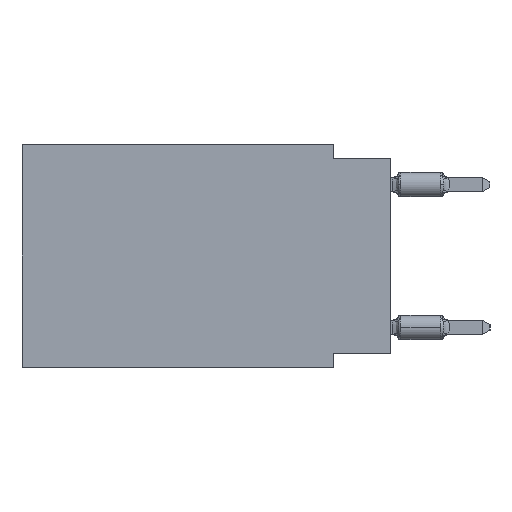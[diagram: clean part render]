
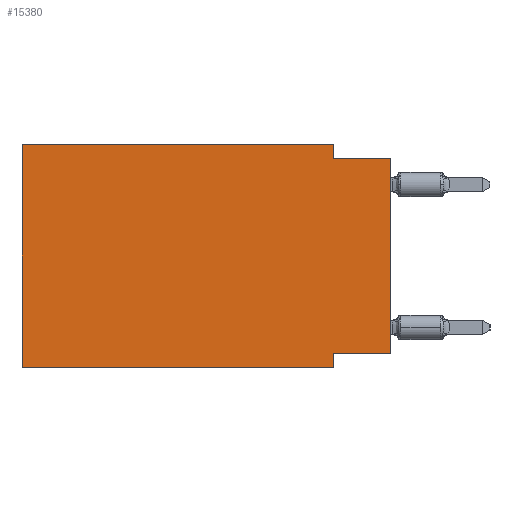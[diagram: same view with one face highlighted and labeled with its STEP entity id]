
A CAD part, left-side view. The second image highlights one B-rep face of the part: STEP entity #15380.
In plain terms, the highlighted planar face has unit normal (-1, 0, 0).
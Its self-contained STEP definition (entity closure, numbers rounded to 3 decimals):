
#7 = CARTESIAN_POINT ( 'NONE',  ( 0., 16.383, 0. ) ) ;
#449 = DIRECTION ( 'NONE',  ( 0., 0., 1. ) ) ;
#732 = CARTESIAN_POINT ( 'NONE',  ( 0., 2.54, -0.635 ) ) ;
#789 = DIRECTION ( 'NONE',  ( 0., -1., 0. ) ) ;
#908 = VECTOR ( 'NONE', #27232, 1000. ) ;
#1753 = VERTEX_POINT ( 'NONE', #9453 ) ;
#2025 = VECTOR ( 'NONE', #2217, 1000. ) ;
#2217 = DIRECTION ( 'NONE',  ( 0., 0., -1. ) ) ;
#2593 = VECTOR ( 'NONE', #26645, 1000. ) ;
#3391 = VECTOR ( 'NONE', #26401, 1000. ) ;
#3669 = VERTEX_POINT ( 'NONE', #732 ) ;
#4281 = EDGE_CURVE ( 'NONE', #1753, #36329, #9491, .T. ) ;
#4875 = CARTESIAN_POINT ( 'NONE',  ( 0., 16.383, 0. ) ) ;
#5067 = FACE_OUTER_BOUND ( 'NONE', #12217, .T. ) ;
#5641 = EDGE_CURVE ( 'NONE', #21608, #11308, #12516, .T. ) ;
#6495 = EDGE_CURVE ( 'NONE', #21608, #1753, #14164, .T. ) ;
#7492 = DIRECTION ( 'NONE',  ( 1., 0., 0. ) ) ;
#8837 = CARTESIAN_POINT ( 'NONE',  ( 0., 0., 0. ) ) ;
#9453 = CARTESIAN_POINT ( 'NONE',  ( 0., 16.383, 0. ) ) ;
#9491 = LINE ( 'NONE', #27344, #24403 ) ;
#10519 = VERTEX_POINT ( 'NONE', #10624 ) ;
#10624 = CARTESIAN_POINT ( 'NONE',  ( 0., 0., -0.635 ) ) ;
#11144 = ORIENTED_EDGE ( 'NONE', *, *, #6495, .F. ) ;
#11308 = VERTEX_POINT ( 'NONE', #15387 ) ;
#12217 = EDGE_LOOP ( 'NONE', ( #23193, #20243, #27697, #16714, #11144, #24544, #30088, #32454 ) ) ;
#12516 = LINE ( 'NONE', #26149, #17912 ) ;
#13715 = AXIS2_PLACEMENT_3D ( 'NONE', #4875, #7492, #21654 ) ;
#14164 = LINE ( 'NONE', #7, #15016 ) ;
#14856 = LINE ( 'NONE', #20455, #3391 ) ;
#14919 = CARTESIAN_POINT ( 'NONE',  ( 0., 0., -9.271 ) ) ;
#15016 = VECTOR ( 'NONE', #19937, 1000. ) ;
#15380 = ADVANCED_FACE ( 'NONE', ( #5067 ), #25196, .F. ) ;
#15387 = CARTESIAN_POINT ( 'NONE',  ( 0., 2.54, -9.906 ) ) ;
#15869 = CARTESIAN_POINT ( 'NONE',  ( 0., 2.54, 0. ) ) ;
#16714 = ORIENTED_EDGE ( 'NONE', *, *, #4281, .F. ) ;
#17912 = VECTOR ( 'NONE', #789, 1000. ) ;
#19282 = EDGE_CURVE ( 'NONE', #35319, #10519, #20199, .T. ) ;
#19937 = DIRECTION ( 'NONE',  ( 0., 0., 1. ) ) ;
#20199 = LINE ( 'NONE', #8837, #36387 ) ;
#20243 = ORIENTED_EDGE ( 'NONE', *, *, #31951, .F. ) ;
#20455 = CARTESIAN_POINT ( 'NONE',  ( 0., 0., -0.635 ) ) ;
#21068 = EDGE_CURVE ( 'NONE', #35319, #33935, #23300, .T. ) ;
#21402 = DIRECTION ( 'NONE',  ( 0., -1., 0. ) ) ;
#21608 = VERTEX_POINT ( 'NONE', #29525 ) ;
#21654 = DIRECTION ( 'NONE',  ( 0., 0., -1. ) ) ;
#22744 = CARTESIAN_POINT ( 'NONE',  ( 0., 2.54, -9.271 ) ) ;
#22899 = LINE ( 'NONE', #31072, #2025 ) ;
#23107 = EDGE_CURVE ( 'NONE', #36329, #3669, #24263, .T. ) ;
#23193 = ORIENTED_EDGE ( 'NONE', *, *, #19282, .T. ) ;
#23300 = LINE ( 'NONE', #14919, #2593 ) ;
#24034 = CARTESIAN_POINT ( 'NONE',  ( 0., 0., -9.271 ) ) ;
#24263 = LINE ( 'NONE', #15869, #908 ) ;
#24403 = VECTOR ( 'NONE', #21402, 1000. ) ;
#24544 = ORIENTED_EDGE ( 'NONE', *, *, #5641, .T. ) ;
#25196 = PLANE ( 'NONE',  #13715 ) ;
#26149 = CARTESIAN_POINT ( 'NONE',  ( 0., 16.383, -9.906 ) ) ;
#26401 = DIRECTION ( 'NONE',  ( 0., -1., 0. ) ) ;
#26645 = DIRECTION ( 'NONE',  ( 0., 1., 0. ) ) ;
#27232 = DIRECTION ( 'NONE',  ( 0., 0., -1. ) ) ;
#27344 = CARTESIAN_POINT ( 'NONE',  ( 0., 16.383, 0. ) ) ;
#27647 = CARTESIAN_POINT ( 'NONE',  ( 0., 2.54, 0. ) ) ;
#27697 = ORIENTED_EDGE ( 'NONE', *, *, #23107, .F. ) ;
#29525 = CARTESIAN_POINT ( 'NONE',  ( 0., 16.383, -9.906 ) ) ;
#30088 = ORIENTED_EDGE ( 'NONE', *, *, #35401, .F. ) ;
#31072 = CARTESIAN_POINT ( 'NONE',  ( 0., 2.54, -9.906 ) ) ;
#31951 = EDGE_CURVE ( 'NONE', #3669, #10519, #14856, .T. ) ;
#32454 = ORIENTED_EDGE ( 'NONE', *, *, #21068, .F. ) ;
#33935 = VERTEX_POINT ( 'NONE', #22744 ) ;
#35319 = VERTEX_POINT ( 'NONE', #24034 ) ;
#35401 = EDGE_CURVE ( 'NONE', #33935, #11308, #22899, .T. ) ;
#36329 = VERTEX_POINT ( 'NONE', #27647 ) ;
#36387 = VECTOR ( 'NONE', #449, 1000. ) ;
